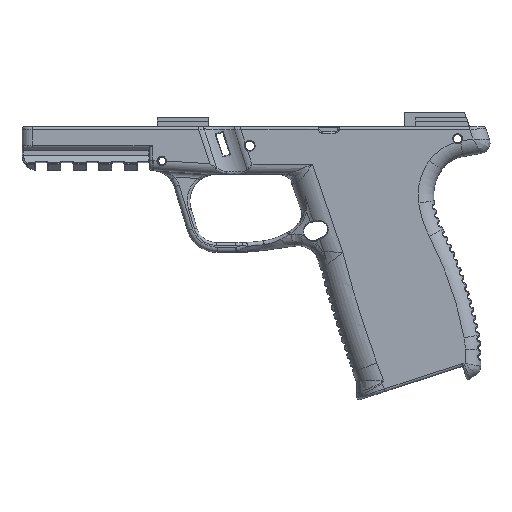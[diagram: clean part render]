
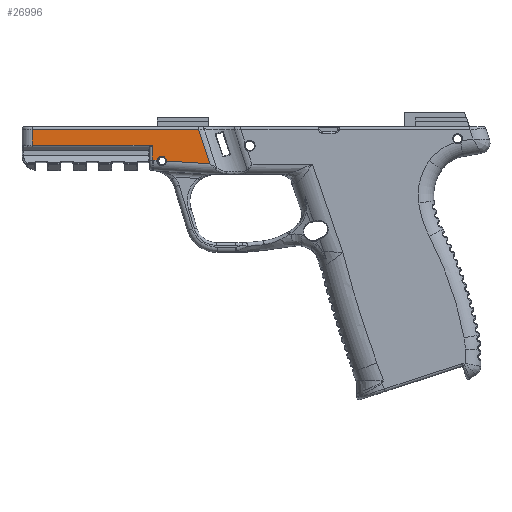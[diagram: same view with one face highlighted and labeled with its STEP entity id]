
A CAD part, top view. The second image highlights one B-rep face of the part: STEP entity #26996.
In plain terms, the highlighted planar face has unit normal (0, 0, 1).
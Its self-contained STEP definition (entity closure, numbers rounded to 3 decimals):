
#321=B_SPLINE_CURVE_WITH_KNOTS('',3,(#41251,#41252,#41253,#41254),
 .UNSPECIFIED.,.F.,.F.,(4,4),(-0.25,-0.249),
 .UNSPECIFIED.);
#323=B_SPLINE_CURVE_WITH_KNOTS('',3,(#41275,#41276,#41277,#41278),
 .UNSPECIFIED.,.F.,.F.,(4,4),(0.249,0.25),
 .UNSPECIFIED.);
#2829=CIRCLE('',#28901,1.838);
#4482=FACE_OUTER_BOUND('',#6280,.T.);
#6280=EDGE_LOOP('',(#18335,#18336,#18337,#18338,#18339,#18340,#18341,#18342,
#18343,#18344,#18345));
#8157=LINE('',#41285,#9638);
#8158=LINE('',#41287,#9639);
#8159=LINE('',#41289,#9640);
#8160=LINE('',#41291,#9641);
#8161=LINE('',#41293,#9642);
#8162=LINE('',#41295,#9643);
#8163=LINE('',#41297,#9644);
#8164=LINE('',#41298,#9645);
#9638=VECTOR('',#32504,10.);
#9639=VECTOR('',#32505,10.);
#9640=VECTOR('',#32506,10.);
#9641=VECTOR('',#32507,10.);
#9642=VECTOR('',#32508,10.);
#9643=VECTOR('',#32509,10.);
#9644=VECTOR('',#32510,10.);
#9645=VECTOR('',#32511,10.);
#11138=VERTEX_POINT('',#41188);
#11141=VERTEX_POINT('',#41207);
#11143=VERTEX_POINT('',#41226);
#11144=VERTEX_POINT('',#41228);
#11147=VERTEX_POINT('',#41284);
#11148=VERTEX_POINT('',#41286);
#11149=VERTEX_POINT('',#41288);
#11150=VERTEX_POINT('',#41290);
#11151=VERTEX_POINT('',#41292);
#11152=VERTEX_POINT('',#41294);
#11153=VERTEX_POINT('',#41296);
#13771=EDGE_CURVE('',#11143,#11144,#2829,.T.);
#13775=EDGE_CURVE('',#11144,#11141,#321,.T.);
#13777=EDGE_CURVE('',#11138,#11143,#323,.T.);
#13779=EDGE_CURVE('',#11147,#11138,#8157,.T.);
#13780=EDGE_CURVE('',#11148,#11147,#8158,.T.);
#13781=EDGE_CURVE('',#11149,#11148,#8159,.T.);
#13782=EDGE_CURVE('',#11150,#11149,#8160,.T.);
#13783=EDGE_CURVE('',#11151,#11150,#8161,.T.);
#13784=EDGE_CURVE('',#11152,#11151,#8162,.T.);
#13785=EDGE_CURVE('',#11153,#11152,#8163,.T.);
#13786=EDGE_CURVE('',#11141,#11153,#8164,.T.);
#18335=ORIENTED_EDGE('',*,*,#13775,.F.);
#18336=ORIENTED_EDGE('',*,*,#13771,.F.);
#18337=ORIENTED_EDGE('',*,*,#13777,.F.);
#18338=ORIENTED_EDGE('',*,*,#13779,.F.);
#18339=ORIENTED_EDGE('',*,*,#13780,.F.);
#18340=ORIENTED_EDGE('',*,*,#13781,.F.);
#18341=ORIENTED_EDGE('',*,*,#13782,.F.);
#18342=ORIENTED_EDGE('',*,*,#13783,.F.);
#18343=ORIENTED_EDGE('',*,*,#13784,.F.);
#18344=ORIENTED_EDGE('',*,*,#13785,.F.);
#18345=ORIENTED_EDGE('',*,*,#13786,.F.);
#26618=PLANE('',#28904);
#26996=ADVANCED_FACE('',(#4482),#26618,.T.);
#28901=AXIS2_PLACEMENT_3D('',#41229,#32495,#32496);
#28904=AXIS2_PLACEMENT_3D('',#41283,#32502,#32503);
#32495=DIRECTION('center_axis',(0.,0.,1.));
#32496=DIRECTION('ref_axis',(1.,0.,0.));
#32502=DIRECTION('center_axis',(0.,0.,1.));
#32503=DIRECTION('ref_axis',(1.,0.,0.));
#32504=DIRECTION('',(-0.998,0.062,0.));
#32505=DIRECTION('',(0.309,-0.951,0.));
#32506=DIRECTION('',(1.,0.,0.));
#32507=DIRECTION('',(0.,1.,0.));
#32508=DIRECTION('',(-1.,0.,0.));
#32509=DIRECTION('',(0.,1.,0.));
#32510=DIRECTION('',(-1.,0.,0.));
#32511=DIRECTION('',(-0.998,0.062,0.));
#41188=CARTESIAN_POINT('',(-28.909,30.458,12.75));
#41207=CARTESIAN_POINT('',(-32.574,30.685,12.75));
#41226=CARTESIAN_POINT('',(-28.909,30.469,12.75));
#41228=CARTESIAN_POINT('',(-32.573,30.696,12.75));
#41229=CARTESIAN_POINT('Origin',(-30.746,30.5,12.75));
#41251=CARTESIAN_POINT('Ctrl Pts',(-32.573,30.696,12.75));
#41252=CARTESIAN_POINT('Ctrl Pts',(-32.573,30.692,12.75));
#41253=CARTESIAN_POINT('Ctrl Pts',(-32.574,30.689,12.75));
#41254=CARTESIAN_POINT('Ctrl Pts',(-32.574,30.685,12.75));
#41275=CARTESIAN_POINT('Ctrl Pts',(-28.909,30.458,12.75));
#41276=CARTESIAN_POINT('Ctrl Pts',(-28.909,30.462,12.75));
#41277=CARTESIAN_POINT('Ctrl Pts',(-28.909,30.466,12.75));
#41278=CARTESIAN_POINT('Ctrl Pts',(-28.909,30.469,12.75));
#41283=CARTESIAN_POINT('Origin',(3.143,-8.368,12.75));
#41284=CARTESIAN_POINT('',(-12.091,29.418,12.75));
#41285=CARTESIAN_POINT('',(-1.92,28.789,12.75));
#41286=CARTESIAN_POINT('',(-16.423,42.75,12.75));
#41287=CARTESIAN_POINT('',(-12.425,30.447,12.75));
#41288=CARTESIAN_POINT('',(-81.,42.75,12.75));
#41289=CARTESIAN_POINT('',(47.696,42.75,12.75));
#41290=CARTESIAN_POINT('',(-81.,36.572,12.75));
#41291=CARTESIAN_POINT('',(-81.,17.691,12.75));
#41292=CARTESIAN_POINT('',(-34.47,36.572,12.75));
#41293=CARTESIAN_POINT('',(-40.929,36.572,12.75));
#41294=CARTESIAN_POINT('',(-34.47,30.758,12.75));
#41295=CARTESIAN_POINT('',(-34.47,9.191,12.75));
#41296=CARTESIAN_POINT('',(-33.75,30.758,12.75));
#41297=CARTESIAN_POINT('',(-33.75,30.758,12.75));
#41298=CARTESIAN_POINT('',(-1.92,28.789,12.75));
